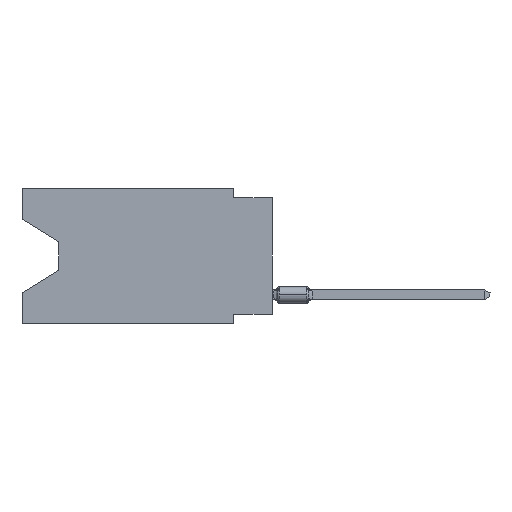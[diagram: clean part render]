
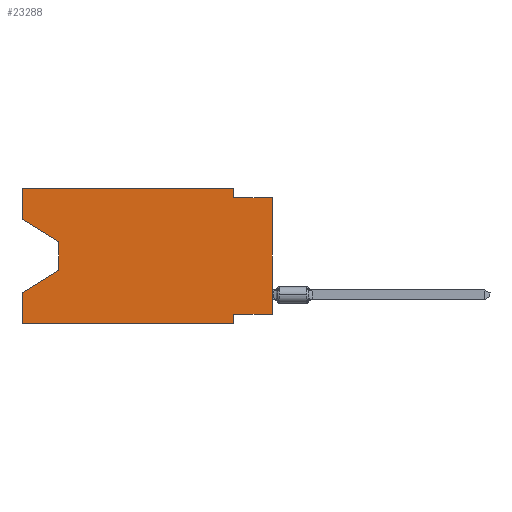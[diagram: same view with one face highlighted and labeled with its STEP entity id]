
A CAD part, left-side view. The second image highlights one B-rep face of the part: STEP entity #23288.
In plain terms, the highlighted planar face has unit normal (-1, 0, 0).
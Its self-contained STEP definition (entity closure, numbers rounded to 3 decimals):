
#179 = CARTESIAN_POINT ( 'NONE',  ( 0., 16.383, 0. ) ) ;
#356 = VECTOR ( 'NONE', #32970, 1000. ) ;
#555 = ORIENTED_EDGE ( 'NONE', *, *, #4379, .F. ) ;
#819 = EDGE_CURVE ( 'NONE', #33862, #8412, #35531, .T. ) ;
#1496 = EDGE_CURVE ( 'NONE', #9789, #2620, #21266, .T. ) ;
#1748 = ORIENTED_EDGE ( 'NONE', *, *, #19070, .T. ) ;
#1765 = CARTESIAN_POINT ( 'NONE',  ( 0., 13.97, -5.385 ) ) ;
#1841 = VERTEX_POINT ( 'NONE', #30764 ) ;
#1857 = EDGE_CURVE ( 'NONE', #30831, #15050, #21714, .T. ) ;
#2148 = CARTESIAN_POINT ( 'NONE',  ( 0., 0., -0.635 ) ) ;
#2554 = VECTOR ( 'NONE', #27132, 1000. ) ;
#2620 = VERTEX_POINT ( 'NONE', #1765 ) ;
#3258 = CARTESIAN_POINT ( 'NONE',  ( 0., 0., 0. ) ) ;
#3627 = CARTESIAN_POINT ( 'NONE',  ( 0., 2.54, -0.635 ) ) ;
#4379 = EDGE_CURVE ( 'NONE', #8412, #28142, #13358, .T. ) ;
#4938 = CARTESIAN_POINT ( 'NONE',  ( 0., 16.383, -8.89 ) ) ;
#4944 = ORIENTED_EDGE ( 'NONE', *, *, #29092, .F. ) ;
#5000 = EDGE_LOOP ( 'NONE', ( #1748, #15054, #15228, #34325, #22996, #27469, #5782, #20306, #23090, #555, #8293, #4944 ) ) ;
#5081 = VERTEX_POINT ( 'NONE', #20169 ) ;
#5782 = ORIENTED_EDGE ( 'NONE', *, *, #8427, .F. ) ;
#7284 = VECTOR ( 'NONE', #24550, 1000. ) ;
#7793 = DIRECTION ( 'NONE',  ( 0., 0., -1. ) ) ;
#7841 = CARTESIAN_POINT ( 'NONE',  ( 0., 2.54, -8.89 ) ) ;
#8059 = CARTESIAN_POINT ( 'NONE',  ( 0., 13.97, -3.505 ) ) ;
#8215 = CARTESIAN_POINT ( 'NONE',  ( 0., 0., -8.255 ) ) ;
#8293 = ORIENTED_EDGE ( 'NONE', *, *, #819, .F. ) ;
#8390 = DIRECTION ( 'NONE',  ( 0., 0., 1. ) ) ;
#8412 = VERTEX_POINT ( 'NONE', #19090 ) ;
#8427 = EDGE_CURVE ( 'NONE', #5081, #24408, #34254, .T. ) ;
#8571 = DIRECTION ( 'NONE',  ( 1., 0., 0. ) ) ;
#8662 = CARTESIAN_POINT ( 'NONE',  ( 0., 16.383, -6.852 ) ) ;
#8765 = DIRECTION ( 'NONE',  ( 0., 0., -1. ) ) ;
#9008 = VECTOR ( 'NONE', #19842, 1000. ) ;
#9316 = CARTESIAN_POINT ( 'NONE',  ( 0., 2.54, -8.89 ) ) ;
#9789 = VERTEX_POINT ( 'NONE', #8059 ) ;
#9803 = LINE ( 'NONE', #32594, #356 ) ;
#10701 = VECTOR ( 'NONE', #34536, 1000. ) ;
#10975 = LINE ( 'NONE', #34145, #10701 ) ;
#11573 = CARTESIAN_POINT ( 'NONE',  ( 0., 13.97, -5.385 ) ) ;
#11715 = CARTESIAN_POINT ( 'NONE',  ( 0., 2.54, -8.255 ) ) ;
#12310 = EDGE_CURVE ( 'NONE', #24408, #32709, #34572, .T. ) ;
#13358 = LINE ( 'NONE', #22275, #35034 ) ;
#13729 = CARTESIAN_POINT ( 'NONE',  ( 0., 16.383, 0. ) ) ;
#14332 = EDGE_CURVE ( 'NONE', #5081, #26199, #34794, .T. ) ;
#15050 = VERTEX_POINT ( 'NONE', #8662 ) ;
#15054 = ORIENTED_EDGE ( 'NONE', *, *, #1496, .T. ) ;
#15073 = VECTOR ( 'NONE', #17500, 1000. ) ;
#15228 = ORIENTED_EDGE ( 'NONE', *, *, #36583, .T. ) ;
#15538 = VECTOR ( 'NONE', #29792, 1000. ) ;
#16471 = VECTOR ( 'NONE', #34947, 1000. ) ;
#16505 = EDGE_CURVE ( 'NONE', #28142, #26199, #21853, .T. ) ;
#17500 = DIRECTION ( 'NONE',  ( 0., 0., -1. ) ) ;
#18605 = CARTESIAN_POINT ( 'NONE',  ( 0., 16.383, -8.89 ) ) ;
#19070 = EDGE_CURVE ( 'NONE', #1841, #9789, #10975, .T. ) ;
#19090 = CARTESIAN_POINT ( 'NONE',  ( 0., 2.54, 0. ) ) ;
#19752 = DIRECTION ( 'NONE',  ( 0., 0.855, -0.519 ) ) ;
#19842 = DIRECTION ( 'NONE',  ( 0., 1., 0. ) ) ;
#19940 = LINE ( 'NONE', #11573, #27083 ) ;
#20169 = CARTESIAN_POINT ( 'NONE',  ( 0., 0., -8.255 ) ) ;
#20306 = ORIENTED_EDGE ( 'NONE', *, *, #14332, .T. ) ;
#21266 = LINE ( 'NONE', #32825, #2554 ) ;
#21714 = LINE ( 'NONE', #28100, #7284 ) ;
#21853 = LINE ( 'NONE', #35721, #26352 ) ;
#22275 = CARTESIAN_POINT ( 'NONE',  ( 0., 2.54, 0. ) ) ;
#22996 = ORIENTED_EDGE ( 'NONE', *, *, #27046, .T. ) ;
#23090 = ORIENTED_EDGE ( 'NONE', *, *, #16505, .F. ) ;
#23288 = ADVANCED_FACE ( 'NONE', ( #28524 ), #25680, .F. ) ;
#24408 = VERTEX_POINT ( 'NONE', #11715 ) ;
#24550 = DIRECTION ( 'NONE',  ( 0., 0., 1. ) ) ;
#25680 = PLANE ( 'NONE',  #27265 ) ;
#26199 = VERTEX_POINT ( 'NONE', #2148 ) ;
#26352 = VECTOR ( 'NONE', #30201, 1000. ) ;
#27046 = EDGE_CURVE ( 'NONE', #30831, #32709, #33017, .T. ) ;
#27083 = VECTOR ( 'NONE', #19752, 1000. ) ;
#27132 = DIRECTION ( 'NONE',  ( 0., 0., -1. ) ) ;
#27265 = AXIS2_PLACEMENT_3D ( 'NONE', #13729, #8571, #8765 ) ;
#27469 = ORIENTED_EDGE ( 'NONE', *, *, #12310, .F. ) ;
#28100 = CARTESIAN_POINT ( 'NONE',  ( 0., 16.383, 0. ) ) ;
#28142 = VERTEX_POINT ( 'NONE', #3627 ) ;
#28524 = FACE_OUTER_BOUND ( 'NONE', #5000, .T. ) ;
#29092 = EDGE_CURVE ( 'NONE', #1841, #33862, #9803, .T. ) ;
#29792 = DIRECTION ( 'NONE',  ( 0., -1., 0. ) ) ;
#30201 = DIRECTION ( 'NONE',  ( 0., -1., 0. ) ) ;
#30764 = CARTESIAN_POINT ( 'NONE',  ( 0., 16.383, -2.038 ) ) ;
#30831 = VERTEX_POINT ( 'NONE', #4938 ) ;
#32124 = VECTOR ( 'NONE', #8390, 1000. ) ;
#32594 = CARTESIAN_POINT ( 'NONE',  ( 0., 16.383, 0. ) ) ;
#32709 = VERTEX_POINT ( 'NONE', #7841 ) ;
#32825 = CARTESIAN_POINT ( 'NONE',  ( 0., 13.97, -3.505 ) ) ;
#32970 = DIRECTION ( 'NONE',  ( 0., 0., 1. ) ) ;
#33017 = LINE ( 'NONE', #18605, #15538 ) ;
#33862 = VERTEX_POINT ( 'NONE', #34468 ) ;
#34145 = CARTESIAN_POINT ( 'NONE',  ( 0., 16.383, -2.038 ) ) ;
#34254 = LINE ( 'NONE', #8215, #9008 ) ;
#34325 = ORIENTED_EDGE ( 'NONE', *, *, #1857, .F. ) ;
#34468 = CARTESIAN_POINT ( 'NONE',  ( 0., 16.383, 0. ) ) ;
#34536 = DIRECTION ( 'NONE',  ( 0., -0.855, -0.519 ) ) ;
#34572 = LINE ( 'NONE', #9316, #15073 ) ;
#34794 = LINE ( 'NONE', #3258, #32124 ) ;
#34947 = DIRECTION ( 'NONE',  ( 0., -1., 0. ) ) ;
#35034 = VECTOR ( 'NONE', #7793, 1000. ) ;
#35531 = LINE ( 'NONE', #179, #16471 ) ;
#35721 = CARTESIAN_POINT ( 'NONE',  ( 0., 0., -0.635 ) ) ;
#36583 = EDGE_CURVE ( 'NONE', #2620, #15050, #19940, .T. ) ;
